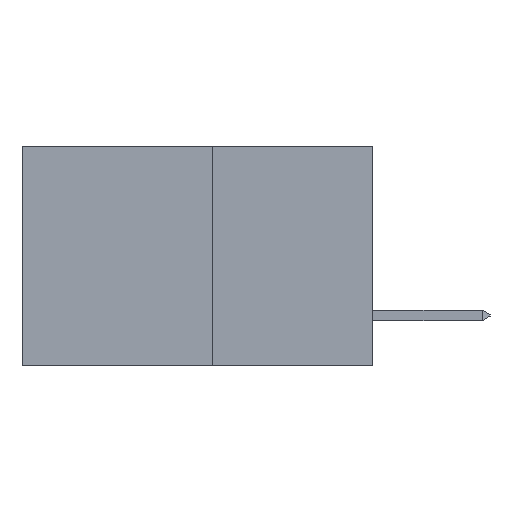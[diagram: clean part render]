
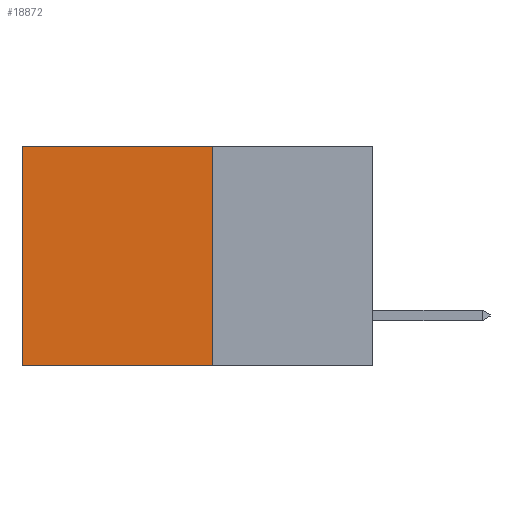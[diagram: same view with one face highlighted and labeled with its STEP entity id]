
A CAD part, left-side view. The second image highlights one B-rep face of the part: STEP entity #18872.
In plain terms, the highlighted planar face has unit normal (-1, 0, 0).
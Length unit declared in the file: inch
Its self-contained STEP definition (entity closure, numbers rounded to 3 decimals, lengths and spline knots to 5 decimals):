
#561 = VECTOR ( 'NONE', #9902, 39.37008 ) ;
#1134 = LINE ( 'NONE', #8130, #561 ) ;
#1315 = DIRECTION ( 'NONE',  ( 1., 0., 0. ) ) ;
#2079 = VERTEX_POINT ( 'NONE', #22575 ) ;
#2105 = AXIS2_PLACEMENT_3D ( 'NONE', #11811, #1315, #13594 ) ;
#2817 = ORIENTED_EDGE ( 'NONE', *, *, #17834, .F. ) ;
#3550 = EDGE_CURVE ( 'NONE', #2079, #9839, #19199, .T. ) ;
#4932 = ORIENTED_EDGE ( 'NONE', *, *, #3550, .F. ) ;
#5204 = VECTOR ( 'NONE', #11284, 39.37008 ) ;
#6744 = DIRECTION ( 'NONE',  ( 0., 0., -1. ) ) ;
#7051 = CARTESIAN_POINT ( 'NONE',  ( 0.277, 0.59, -0.37 ) ) ;
#8130 = CARTESIAN_POINT ( 'NONE',  ( 0.277, 0.27, 0. ) ) ;
#9839 = VERTEX_POINT ( 'NONE', #11705 ) ;
#9855 = FACE_OUTER_BOUND ( 'NONE', #19113, .T. ) ;
#9902 = DIRECTION ( 'NONE',  ( 0., 1., 0. ) ) ;
#10194 = ORIENTED_EDGE ( 'NONE', *, *, #14948, .T. ) ;
#11284 = DIRECTION ( 'NONE',  ( 0., 0., -1. ) ) ;
#11705 = CARTESIAN_POINT ( 'NONE',  ( 0.277, 0.27, -0.37 ) ) ;
#11811 = CARTESIAN_POINT ( 'NONE',  ( 0.277, 0.27, -0.37 ) ) ;
#12296 = CARTESIAN_POINT ( 'NONE',  ( 0.277, 0.27, -0.37 ) ) ;
#13594 = DIRECTION ( 'NONE',  ( 0., 0., -1. ) ) ;
#13749 = CARTESIAN_POINT ( 'NONE',  ( 0.277, 0.59, -0.37 ) ) ;
#14081 = DIRECTION ( 'NONE',  ( 0., 1., 0. ) ) ;
#14236 = EDGE_CURVE ( 'NONE', #2079, #16203, #1134, .T. ) ;
#14948 = EDGE_CURVE ( 'NONE', #16203, #21980, #21046, .T. ) ;
#16203 = VERTEX_POINT ( 'NONE', #18831 ) ;
#16377 = VECTOR ( 'NONE', #6744, 39.37008 ) ;
#17834 = EDGE_CURVE ( 'NONE', #9839, #21980, #19524, .T. ) ;
#18434 = VECTOR ( 'NONE', #14081, 39.37008 ) ;
#18831 = CARTESIAN_POINT ( 'NONE',  ( 0.277, 0.59, 0. ) ) ;
#18872 = ADVANCED_FACE ( 'NONE', ( #9855 ), #22341, .F. ) ;
#19113 = EDGE_LOOP ( 'NONE', ( #10194, #2817, #4932, #20727 ) ) ;
#19199 = LINE ( 'NONE', #19440, #5204 ) ;
#19440 = CARTESIAN_POINT ( 'NONE',  ( 0.277, 0.27, -0.37 ) ) ;
#19524 = LINE ( 'NONE', #12296, #18434 ) ;
#20727 = ORIENTED_EDGE ( 'NONE', *, *, #14236, .T. ) ;
#21046 = LINE ( 'NONE', #13749, #16377 ) ;
#21980 = VERTEX_POINT ( 'NONE', #7051 ) ;
#22341 = PLANE ( 'NONE',  #2105 ) ;
#22575 = CARTESIAN_POINT ( 'NONE',  ( 0.277, 0.27, 0. ) ) ;
